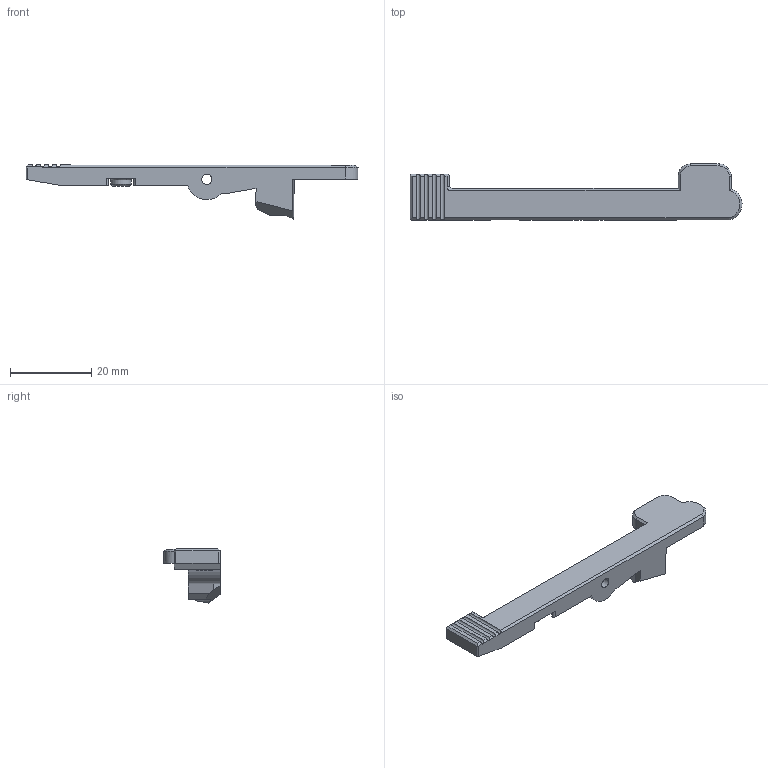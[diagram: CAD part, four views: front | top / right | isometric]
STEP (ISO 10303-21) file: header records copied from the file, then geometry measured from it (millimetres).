
FILE_DESCRIPTION (( 'STEP AP203' ), '1' );
FILE_NAME ('MOD9_V3_Mag_Release.STEP', '2020-12-23T19:11:35', ( '' ), ( '' ), 'SwSTEP 2.0', 'SolidWorks 2019', '' );
FILE_SCHEMA (( 'CONFIG_CONTROL_DESIGN' ));
Length unit declared in the file: millimetre
Products named in the file (1): MOD9_V3_Mag_Release
Bounding box: 81.77 x 13.8 x 13.32 mm (x, y, z)
Volume: 3876.3 mm3; surface area: 2683.5 mm2
Topology: 1 solids, 1 shells, 81 faces, 217 edges, 139 vertices
Faces by surface type: plane 48, cylinder 26, cone 5, bspline 2
Entity records: 2660 total; most frequent: CARTESIAN_POINT 662, ORIENTED_EDGE 434, DIRECTION 363, EDGE_CURVE 217, VECTOR 143, LINE 143, VERTEX_POINT 139, AXIS2_PLACEMENT_3D 110
